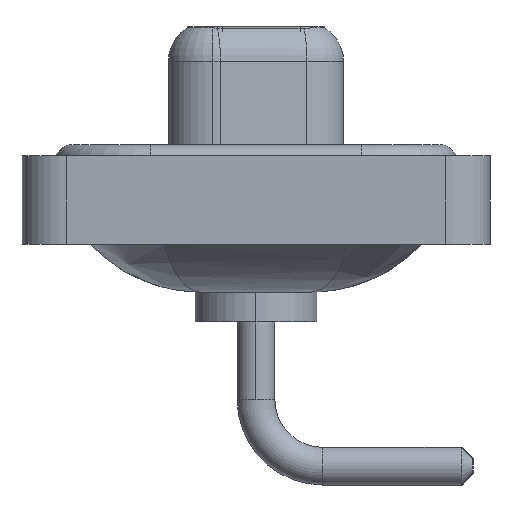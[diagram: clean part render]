
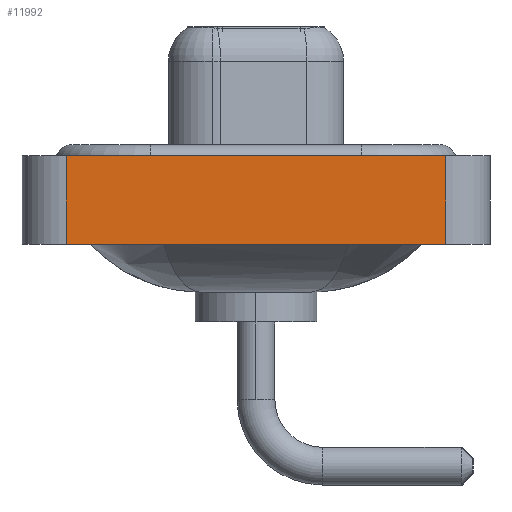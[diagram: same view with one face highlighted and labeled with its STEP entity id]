
A CAD part, left-side view. The second image highlights one B-rep face of the part: STEP entity #11992.
In plain terms, the highlighted planar face has unit normal (-1, 0, 0).
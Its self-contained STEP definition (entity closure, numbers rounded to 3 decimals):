
#407 = LINE ( 'NONE', #752, #16428 ) ;
#752 = CARTESIAN_POINT ( 'NONE',  ( -7.3, 8.55, -3.6 ) ) ;
#1104 = ORIENTED_EDGE ( 'NONE', *, *, #15700, .T. ) ;
#2089 = CARTESIAN_POINT ( 'NONE',  ( -7.3, -8.55, -3.6 ) ) ;
#3232 = DIRECTION ( 'NONE',  ( 0., -1., 0. ) ) ;
#3403 = CARTESIAN_POINT ( 'NONE',  ( -7.3, -8.55, -3.6 ) ) ;
#3656 = FACE_OUTER_BOUND ( 'NONE', #11117, .T. ) ;
#4340 = VERTEX_POINT ( 'NONE', #4894 ) ;
#4804 = DIRECTION ( 'NONE',  ( 0., 0., 1. ) ) ;
#4820 = LINE ( 'NONE', #16019, #10024 ) ;
#4894 = CARTESIAN_POINT ( 'NONE',  ( -7.3, 8.55, 0.4 ) ) ;
#5078 = PLANE ( 'NONE',  #7349 ) ;
#5420 = VECTOR ( 'NONE', #4804, 1000. ) ;
#6715 = VERTEX_POINT ( 'NONE', #6969 ) ;
#6969 = CARTESIAN_POINT ( 'NONE',  ( -7.3, -8.55, 0.4 ) ) ;
#7192 = CARTESIAN_POINT ( 'NONE',  ( -7.3, -8.55, -3.6 ) ) ;
#7275 = VERTEX_POINT ( 'NONE', #3403 ) ;
#7349 = AXIS2_PLACEMENT_3D ( 'NONE', #10495, #9072, #13246 ) ;
#7698 = EDGE_CURVE ( 'NONE', #10083, #4340, #407, .T. ) ;
#7746 = EDGE_CURVE ( 'NONE', #7275, #6715, #8519, .T. ) ;
#8408 = VECTOR ( 'NONE', #3232, 1000. ) ;
#8519 = LINE ( 'NONE', #7192, #5420 ) ;
#8729 = ORIENTED_EDGE ( 'NONE', *, *, #9417, .F. ) ;
#9072 = DIRECTION ( 'NONE',  ( -1., 0., 0. ) ) ;
#9417 = EDGE_CURVE ( 'NONE', #4340, #6715, #4820, .T. ) ;
#10024 = VECTOR ( 'NONE', #11999, 1000. ) ;
#10083 = VERTEX_POINT ( 'NONE', #12544 ) ;
#10495 = CARTESIAN_POINT ( 'NONE',  ( -7.3, -8.55, -3.6 ) ) ;
#11117 = EDGE_LOOP ( 'NONE', ( #16632, #8729, #16829, #1104 ) ) ;
#11992 = ADVANCED_FACE ( 'NONE', ( #3656 ), #5078, .T. ) ;
#11999 = DIRECTION ( 'NONE',  ( 0., -1., 0. ) ) ;
#12544 = CARTESIAN_POINT ( 'NONE',  ( -7.3, 8.55, -3.6 ) ) ;
#12617 = DIRECTION ( 'NONE',  ( 0., 0., 1. ) ) ;
#13246 = DIRECTION ( 'NONE',  ( 0., 0., 1. ) ) ;
#14226 = LINE ( 'NONE', #2089, #8408 ) ;
#15700 = EDGE_CURVE ( 'NONE', #10083, #7275, #14226, .T. ) ;
#16019 = CARTESIAN_POINT ( 'NONE',  ( -7.3, -8.55, 0.4 ) ) ;
#16428 = VECTOR ( 'NONE', #12617, 1000. ) ;
#16632 = ORIENTED_EDGE ( 'NONE', *, *, #7746, .T. ) ;
#16829 = ORIENTED_EDGE ( 'NONE', *, *, #7698, .F. ) ;
